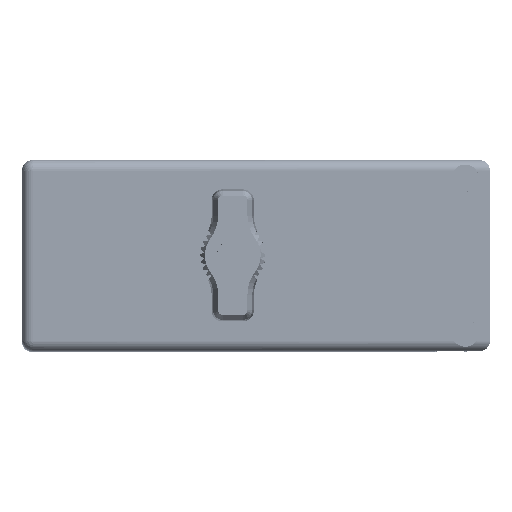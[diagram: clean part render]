
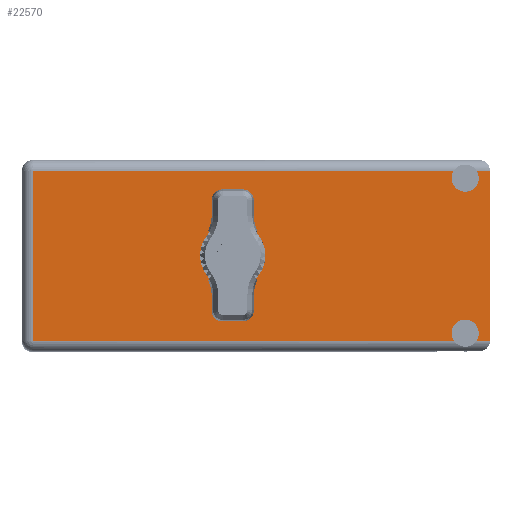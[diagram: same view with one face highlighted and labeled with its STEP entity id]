
A CAD part, top view. The second image highlights one B-rep face of the part: STEP entity #22570.
In plain terms, the highlighted face is planar.
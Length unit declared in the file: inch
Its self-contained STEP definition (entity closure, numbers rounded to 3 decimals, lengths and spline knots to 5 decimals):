
#172 = DIRECTION ( 'NONE',  ( -1., 0., 0. ) ) ;
#759 = CARTESIAN_POINT ( 'NONE',  ( 0., 1.675, 0.125 ) ) ;
#1102 = VECTOR ( 'NONE', #49334, 39.37008 ) ;
#2121 = VECTOR ( 'NONE', #172, 39.37008 ) ;
#3444 = DIRECTION ( 'NONE',  ( 0., 1., 0. ) ) ;
#4146 = CARTESIAN_POINT ( 'NONE',  ( 1.499, 1.675, 0.5 ) ) ;
#4397 = DIRECTION ( 'NONE',  ( 0., 1., 0. ) ) ;
#5763 = CARTESIAN_POINT ( 'NONE',  ( 1.659, 1.675, 0.547 ) ) ;
#6682 = DIRECTION ( 'NONE',  ( -1., 0., 0. ) ) ;
#8865 = VERTEX_POINT ( 'NONE', #26444 ) ;
#9204 = EDGE_CURVE ( 'NONE', #15421, #78058, #76442, .T. ) ;
#9294 = CARTESIAN_POINT ( 'NONE',  ( 1.42519, 1.675, -0.547 ) ) ;
#11651 = LINE ( 'NONE', #93906, #1102 ) ;
#11662 = DIRECTION ( 'NONE',  ( 0., 0., 1. ) ) ;
#11737 = AXIS2_PLACEMENT_3D ( 'NONE', #31254, #38427, #60924 ) ;
#11756 = VERTEX_POINT ( 'NONE', #20165 ) ;
#11895 = DIRECTION ( 'NONE',  ( 0., 0., 1. ) ) ;
#13826 = ORIENTED_EDGE ( 'NONE', *, *, #80210, .F. ) ;
#13875 = VERTEX_POINT ( 'NONE', #47263 ) ;
#14413 = ORIENTED_EDGE ( 'NONE', *, *, #77660, .F. ) ;
#15421 = VERTEX_POINT ( 'NONE', #21332 ) ;
#17292 = VERTEX_POINT ( 'NONE', #9294 ) ;
#17297 = LINE ( 'NONE', #38115, #2121 ) ;
#17774 = CARTESIAN_POINT ( 'NONE',  ( -1.289, 1.675, 0.547 ) ) ;
#19238 = ORIENTED_EDGE ( 'NONE', *, *, #82642, .T. ) ;
#20164 = AXIS2_PLACEMENT_3D ( 'NONE', #93781, #4397, #11895 ) ;
#20165 = CARTESIAN_POINT ( 'NONE',  ( 1.659, 1.675, 0.547 ) ) ;
#20226 = EDGE_CURVE ( 'NONE', #8865, #50882, #70070, .T. ) ;
#20607 = DIRECTION ( 'NONE',  ( 0., 0., 1. ) ) ;
#21332 = CARTESIAN_POINT ( 'NONE',  ( 0., 1.675, -0.125 ) ) ;
#21628 = ORIENTED_EDGE ( 'NONE', *, *, #69282, .F. ) ;
#21940 = CIRCLE ( 'NONE', #66922, 0.0875 ) ;
#22570 = ADVANCED_FACE ( 'NONE', ( #79116, #57048 ), #32923, .T. ) ;
#25007 = CARTESIAN_POINT ( 'NONE',  ( -1.359, 1.675, -0.617 ) ) ;
#26444 = CARTESIAN_POINT ( 'NONE',  ( -1.289, 1.675, -0.547 ) ) ;
#27230 = CARTESIAN_POINT ( 'NONE',  ( 1.499, 1.675, -0.4125 ) ) ;
#31254 = CARTESIAN_POINT ( 'NONE',  ( 0., 1.675, 0. ) ) ;
#31965 = LINE ( 'NONE', #80191, #38992 ) ;
#32923 = PLANE ( 'NONE',  #91130 ) ;
#33661 = EDGE_CURVE ( 'NONE', #78058, #15421, #94249, .T. ) ;
#33860 = ORIENTED_EDGE ( 'NONE', *, *, #33661, .F. ) ;
#36182 = ORIENTED_EDGE ( 'NONE', *, *, #79579, .T. ) ;
#38115 = CARTESIAN_POINT ( 'NONE',  ( -1.359, 1.675, -0.547 ) ) ;
#38427 = DIRECTION ( 'NONE',  ( 0., 1., 0. ) ) ;
#38992 = VECTOR ( 'NONE', #69335, 39.37008 ) ;
#39166 = CIRCLE ( 'NONE', #62176, 0.0875 ) ;
#39773 = CIRCLE ( 'NONE', #66944, 0.0875 ) ;
#40246 = VECTOR ( 'NONE', #87306, 39.37008 ) ;
#40885 = VERTEX_POINT ( 'NONE', #27230 ) ;
#41617 = ORIENTED_EDGE ( 'NONE', *, *, #62157, .T. ) ;
#42586 = CARTESIAN_POINT ( 'NONE',  ( 1.499, 1.675, 0.5 ) ) ;
#43665 = DIRECTION ( 'NONE',  ( 0., 1., 0. ) ) ;
#43928 = EDGE_LOOP ( 'NONE', ( #33860, #87328 ) ) ;
#43974 = DIRECTION ( 'NONE',  ( 0., 0., 1. ) ) ;
#43985 = CARTESIAN_POINT ( 'NONE',  ( -1.359, 1.675, -0.547 ) ) ;
#44368 = VERTEX_POINT ( 'NONE', #67829 ) ;
#44492 = VERTEX_POINT ( 'NONE', #62921 ) ;
#47263 = CARTESIAN_POINT ( 'NONE',  ( 1.57281, 1.675, 0.547 ) ) ;
#47620 = DIRECTION ( 'NONE',  ( -1., 0., 0. ) ) ;
#49288 = ORIENTED_EDGE ( 'NONE', *, *, #64851, .T. ) ;
#49334 = DIRECTION ( 'NONE',  ( 1., 0., 0. ) ) ;
#50882 = VERTEX_POINT ( 'NONE', #17774 ) ;
#57048 = FACE_OUTER_BOUND ( 'NONE', #88753, .T. ) ;
#59496 = ORIENTED_EDGE ( 'NONE', *, *, #96274, .F. ) ;
#60924 = DIRECTION ( 'NONE',  ( 0., 0., 1. ) ) ;
#61179 = CARTESIAN_POINT ( 'NONE',  ( 1.42519, 1.675, 0.547 ) ) ;
#62157 = EDGE_CURVE ( 'NONE', #17292, #8865, #17297, .T. ) ;
#62176 = AXIS2_PLACEMENT_3D ( 'NONE', #42586, #79961, #20607 ) ;
#62921 = CARTESIAN_POINT ( 'NONE',  ( 1.659, 1.675, -0.547 ) ) ;
#64851 = EDGE_CURVE ( 'NONE', #13875, #11756, #11651, .T. ) ;
#66922 = AXIS2_PLACEMENT_3D ( 'NONE', #80484, #81141, #73642 ) ;
#66944 = AXIS2_PLACEMENT_3D ( 'NONE', #4146, #86971, #71062 ) ;
#67829 = CARTESIAN_POINT ( 'NONE',  ( 1.499, 1.675, 0.4125 ) ) ;
#68138 = ORIENTED_EDGE ( 'NONE', *, *, #20226, .T. ) ;
#68830 = VECTOR ( 'NONE', #11662, 39.37008 ) ;
#69282 = EDGE_CURVE ( 'NONE', #44492, #11756, #31965, .T. ) ;
#69335 = DIRECTION ( 'NONE',  ( 0., 0., 1. ) ) ;
#70070 = LINE ( 'NONE', #93869, #68830 ) ;
#71062 = DIRECTION ( 'NONE',  ( 0., 0., 1. ) ) ;
#72930 = CARTESIAN_POINT ( 'NONE',  ( 0., 1.675, 0. ) ) ;
#73595 = VERTEX_POINT ( 'NONE', #82465 ) ;
#73642 = DIRECTION ( 'NONE',  ( 0., 0., 1. ) ) ;
#76442 = CIRCLE ( 'NONE', #82106, 0.125 ) ;
#77660 = EDGE_CURVE ( 'NONE', #13875, #44368, #39773, .T. ) ;
#78058 = VERTEX_POINT ( 'NONE', #759 ) ;
#79116 = FACE_BOUND ( 'NONE', #43928, .T. ) ;
#79579 = EDGE_CURVE ( 'NONE', #44492, #73595, #80242, .T. ) ;
#79716 = VERTEX_POINT ( 'NONE', #61179 ) ;
#79961 = DIRECTION ( 'NONE',  ( 0., 1., 0. ) ) ;
#80191 = CARTESIAN_POINT ( 'NONE',  ( 1.659, 1.675, 0.617 ) ) ;
#80210 = EDGE_CURVE ( 'NONE', #40885, #73595, #93026, .T. ) ;
#80242 = LINE ( 'NONE', #43985, #81476 ) ;
#80484 = CARTESIAN_POINT ( 'NONE',  ( 1.499, 1.675, -0.5 ) ) ;
#81141 = DIRECTION ( 'NONE',  ( 0., 1., 0. ) ) ;
#81476 = VECTOR ( 'NONE', #6682, 39.37008 ) ;
#82106 = AXIS2_PLACEMENT_3D ( 'NONE', #72930, #43665, #43974 ) ;
#82465 = CARTESIAN_POINT ( 'NONE',  ( 1.57281, 1.675, -0.547 ) ) ;
#82642 = EDGE_CURVE ( 'NONE', #50882, #79716, #93779, .T. ) ;
#86971 = DIRECTION ( 'NONE',  ( 0., 1., 0. ) ) ;
#87306 = DIRECTION ( 'NONE',  ( 1., 0., 0. ) ) ;
#87328 = ORIENTED_EDGE ( 'NONE', *, *, #9204, .F. ) ;
#88511 = EDGE_CURVE ( 'NONE', #17292, #40885, #21940, .T. ) ;
#88753 = EDGE_LOOP ( 'NONE', ( #19238, #59496, #14413, #49288, #21628, #36182, #13826, #90540, #41617, #68138 ) ) ;
#90540 = ORIENTED_EDGE ( 'NONE', *, *, #88511, .F. ) ;
#91130 = AXIS2_PLACEMENT_3D ( 'NONE', #25007, #3444, #47620 ) ;
#93026 = CIRCLE ( 'NONE', #20164, 0.0875 ) ;
#93779 = LINE ( 'NONE', #5763, #40246 ) ;
#93781 = CARTESIAN_POINT ( 'NONE',  ( 1.499, 1.675, -0.5 ) ) ;
#93869 = CARTESIAN_POINT ( 'NONE',  ( -1.289, 1.675, -0.617 ) ) ;
#93906 = CARTESIAN_POINT ( 'NONE',  ( 1.659, 1.675, 0.547 ) ) ;
#94249 = CIRCLE ( 'NONE', #11737, 0.125 ) ;
#96274 = EDGE_CURVE ( 'NONE', #44368, #79716, #39166, .T. ) ;
